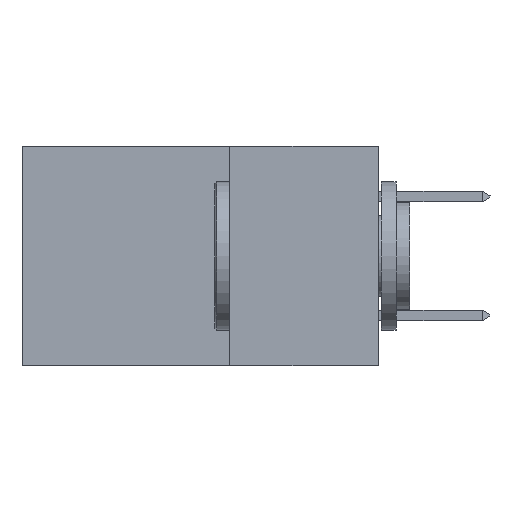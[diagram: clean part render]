
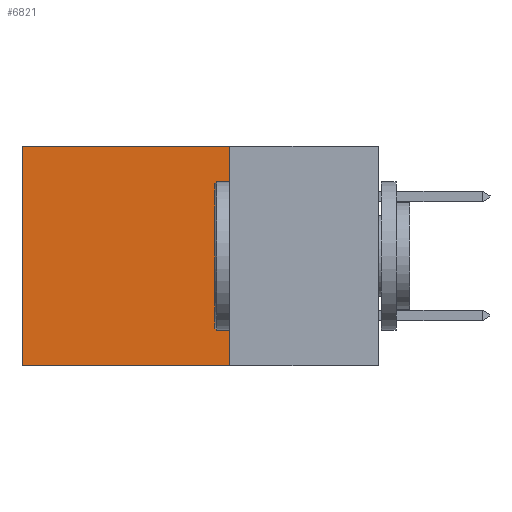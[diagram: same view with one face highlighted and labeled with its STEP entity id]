
A CAD part, left-side view. The second image highlights one B-rep face of the part: STEP entity #6821.
In plain terms, the highlighted planar face has unit normal (-1, 0, 0).
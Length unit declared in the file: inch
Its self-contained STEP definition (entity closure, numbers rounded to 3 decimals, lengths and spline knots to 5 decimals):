
#127 = CARTESIAN_POINT ( 'NONE',  ( 0.2615, 0.25, -0.37 ) ) ;
#369 = DIRECTION ( 'NONE',  ( 0., 0., -1. ) ) ;
#1207 = EDGE_CURVE ( 'NONE', #5552, #14810, #14005, .T. ) ;
#2180 = VERTEX_POINT ( 'NONE', #5566 ) ;
#2528 = DIRECTION ( 'NONE',  ( 1., 0., 0. ) ) ;
#2687 = CARTESIAN_POINT ( 'NONE',  ( 0.2615, 0.25, 0. ) ) ;
#2982 = AXIS2_PLACEMENT_3D ( 'NONE', #127, #2528, #12745 ) ;
#5380 = FACE_OUTER_BOUND ( 'NONE', #10887, .T. ) ;
#5552 = VERTEX_POINT ( 'NONE', #2687 ) ;
#5566 = CARTESIAN_POINT ( 'NONE',  ( 0.2615, 0.6, -0.37 ) ) ;
#6553 = ORIENTED_EDGE ( 'NONE', *, *, #16313, .T. ) ;
#6821 = ADVANCED_FACE ( 'NONE', ( #5380 ), #11561, .F. ) ;
#7087 = CARTESIAN_POINT ( 'NONE',  ( 0.2615, 0.6, 0. ) ) ;
#8634 = VECTOR ( 'NONE', #11318, 39.37008 ) ;
#9449 = CARTESIAN_POINT ( 'NONE',  ( 0.2615, 0.25, -0.37 ) ) ;
#9591 = CARTESIAN_POINT ( 'NONE',  ( 0.2615, 0.25, -0.37 ) ) ;
#9928 = CARTESIAN_POINT ( 'NONE',  ( 0.2615, 0.6, -0.37 ) ) ;
#10301 = LINE ( 'NONE', #15409, #15531 ) ;
#10887 = EDGE_LOOP ( 'NONE', ( #6553, #15735, #12909, #16323 ) ) ;
#11247 = VECTOR ( 'NONE', #13551, 39.37008 ) ;
#11318 = DIRECTION ( 'NONE',  ( 0., 1., 0. ) ) ;
#11561 = PLANE ( 'NONE',  #2982 ) ;
#11741 = VECTOR ( 'NONE', #12360, 39.37008 ) ;
#12360 = DIRECTION ( 'NONE',  ( 0., 0., -1. ) ) ;
#12745 = DIRECTION ( 'NONE',  ( 0., 0., -1. ) ) ;
#12909 = ORIENTED_EDGE ( 'NONE', *, *, #12937, .F. ) ;
#12937 = EDGE_CURVE ( 'NONE', #5552, #14842, #10301, .T. ) ;
#13551 = DIRECTION ( 'NONE',  ( 0., 1., 0. ) ) ;
#13729 = LINE ( 'NONE', #9928, #11741 ) ;
#14005 = LINE ( 'NONE', #14166, #8634 ) ;
#14166 = CARTESIAN_POINT ( 'NONE',  ( 0.2615, 0.25, 0. ) ) ;
#14810 = VERTEX_POINT ( 'NONE', #7087 ) ;
#14828 = EDGE_CURVE ( 'NONE', #14842, #2180, #15952, .T. ) ;
#14842 = VERTEX_POINT ( 'NONE', #9591 ) ;
#15409 = CARTESIAN_POINT ( 'NONE',  ( 0.2615, 0.25, -0.37 ) ) ;
#15531 = VECTOR ( 'NONE', #369, 39.37008 ) ;
#15735 = ORIENTED_EDGE ( 'NONE', *, *, #14828, .F. ) ;
#15952 = LINE ( 'NONE', #9449, #11247 ) ;
#16313 = EDGE_CURVE ( 'NONE', #14810, #2180, #13729, .T. ) ;
#16323 = ORIENTED_EDGE ( 'NONE', *, *, #1207, .T. ) ;
